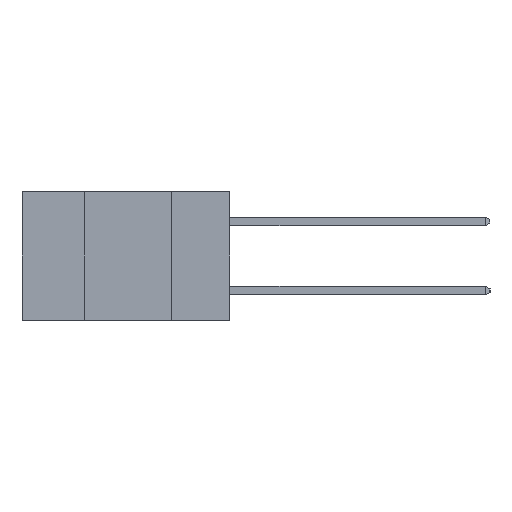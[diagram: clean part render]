
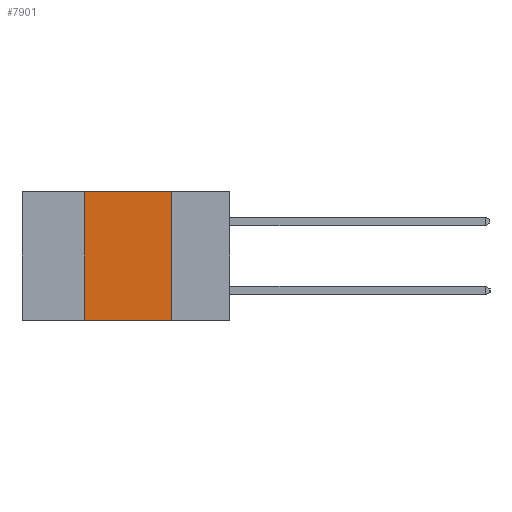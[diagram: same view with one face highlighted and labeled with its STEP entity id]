
A CAD part, left-side view. The second image highlights one B-rep face of the part: STEP entity #7901.
In plain terms, the highlighted planar face has unit normal (-1, 0, 0).
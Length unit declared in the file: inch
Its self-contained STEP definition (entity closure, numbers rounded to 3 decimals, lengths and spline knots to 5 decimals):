
#13 = DIRECTION ( 'NONE',  ( 1., 0., 0. ) ) ;
#77 = CARTESIAN_POINT ( 'NONE',  ( 0., 0.42, -0.37 ) ) ;
#140 = CARTESIAN_POINT ( 'NONE',  ( 0., 0.6, 0. ) ) ;
#179 = PLANE ( 'NONE',  #3610 ) ;
#489 = LINE ( 'NONE', #5426, #3811 ) ;
#596 = DIRECTION ( 'NONE',  ( 0., 0., -1. ) ) ;
#865 = ORIENTED_EDGE ( 'NONE', *, *, #905, .F. ) ;
#905 = EDGE_CURVE ( 'NONE', #8711, #10176, #2118, .T. ) ;
#1179 = VECTOR ( 'NONE', #11976, 39.37008 ) ;
#1840 = CARTESIAN_POINT ( 'NONE',  ( 0., 0.17, 0. ) ) ;
#2118 = LINE ( 'NONE', #13706, #14855 ) ;
#2615 = ORIENTED_EDGE ( 'NONE', *, *, #3929, .T. ) ;
#3465 = EDGE_CURVE ( 'NONE', #12466, #13686, #489, .T. ) ;
#3610 = AXIS2_PLACEMENT_3D ( 'NONE', #140, #13, #15811 ) ;
#3811 = VECTOR ( 'NONE', #5904, 39.37008 ) ;
#3929 = EDGE_CURVE ( 'NONE', #12466, #10176, #13687, .T. ) ;
#4125 = LINE ( 'NONE', #12060, #1179 ) ;
#5426 = CARTESIAN_POINT ( 'NONE',  ( 0., 0.42, -0.37 ) ) ;
#5904 = DIRECTION ( 'NONE',  ( 0., 0., 1. ) ) ;
#6222 = CARTESIAN_POINT ( 'NONE',  ( 0., 0.17, -0.37 ) ) ;
#6720 = EDGE_LOOP ( 'NONE', ( #865, #8066, #15287, #2615 ) ) ;
#7452 = CARTESIAN_POINT ( 'NONE',  ( 0., 0.42, 0. ) ) ;
#7795 = FACE_OUTER_BOUND ( 'NONE', #6720, .T. ) ;
#7901 = ADVANCED_FACE ( 'NONE', ( #7795 ), #179, .F. ) ;
#8066 = ORIENTED_EDGE ( 'NONE', *, *, #13277, .F. ) ;
#8711 = VERTEX_POINT ( 'NONE', #1840 ) ;
#9844 = DIRECTION ( 'NONE',  ( 0., -1., 0. ) ) ;
#10004 = CARTESIAN_POINT ( 'NONE',  ( 0., 0.6, -0.37 ) ) ;
#10039 = VECTOR ( 'NONE', #9844, 39.37008 ) ;
#10176 = VERTEX_POINT ( 'NONE', #6222 ) ;
#11976 = DIRECTION ( 'NONE',  ( 0., -1., 0. ) ) ;
#12060 = CARTESIAN_POINT ( 'NONE',  ( 0., 0.6, 0. ) ) ;
#12466 = VERTEX_POINT ( 'NONE', #77 ) ;
#13277 = EDGE_CURVE ( 'NONE', #13686, #8711, #4125, .T. ) ;
#13686 = VERTEX_POINT ( 'NONE', #7452 ) ;
#13687 = LINE ( 'NONE', #10004, #10039 ) ;
#13706 = CARTESIAN_POINT ( 'NONE',  ( 0., 0.17, -0.37 ) ) ;
#14855 = VECTOR ( 'NONE', #596, 39.37008 ) ;
#15287 = ORIENTED_EDGE ( 'NONE', *, *, #3465, .F. ) ;
#15811 = DIRECTION ( 'NONE',  ( 0., 0., -1. ) ) ;
